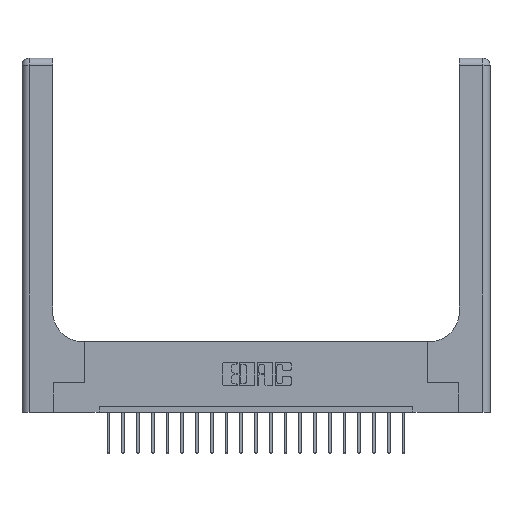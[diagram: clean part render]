
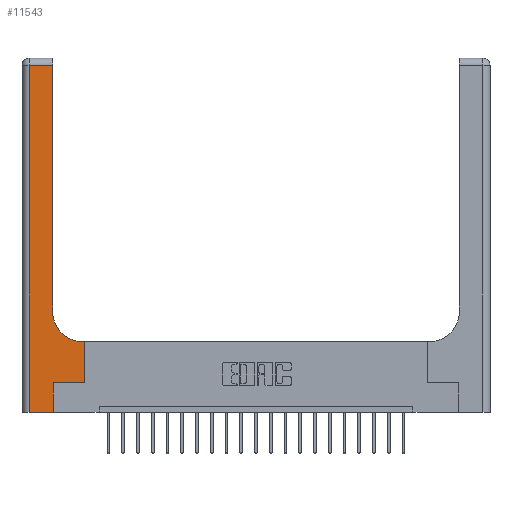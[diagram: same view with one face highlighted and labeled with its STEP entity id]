
A CAD part, top view. The second image highlights one B-rep face of the part: STEP entity #11543.
In plain terms, the highlighted planar face has unit normal (0, 0, 1).
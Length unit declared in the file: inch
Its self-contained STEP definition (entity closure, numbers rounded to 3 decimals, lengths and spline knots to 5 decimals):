
#405 = ORIENTED_EDGE ( 'NONE', *, *, #6993, .T. ) ;
#1041 = CARTESIAN_POINT ( 'NONE',  ( 0.26, 2.94, 0.37 ) ) ;
#1133 = EDGE_CURVE ( 'NONE', #8894, #18805, #10261, .T. ) ;
#1450 = VERTEX_POINT ( 'NONE', #1041 ) ;
#1686 = DIRECTION ( 'NONE',  ( 0., 1., 0. ) ) ;
#1790 = FACE_OUTER_BOUND ( 'NONE', #7415, .T. ) ;
#1892 = DIRECTION ( 'NONE',  ( 0., 0., -1. ) ) ;
#2078 = EDGE_CURVE ( 'NONE', #5481, #1450, #10321, .T. ) ;
#2083 = VECTOR ( 'NONE', #10715, 39.37008 ) ;
#2182 = EDGE_CURVE ( 'NONE', #18805, #15296, #10542, .T. ) ;
#2325 = LINE ( 'NONE', #15711, #11010 ) ;
#2401 = CARTESIAN_POINT ( 'NONE',  ( 0.26, 3., 0.37 ) ) ;
#2431 = LINE ( 'NONE', #17546, #16865 ) ;
#2942 = ORIENTED_EDGE ( 'NONE', *, *, #8634, .T. ) ;
#3044 = EDGE_CURVE ( 'NONE', #15296, #12000, #2431, .T. ) ;
#3555 = CARTESIAN_POINT ( 'NONE',  ( 0., 0., 0.37 ) ) ;
#3793 = ORIENTED_EDGE ( 'NONE', *, *, #3044, .T. ) ;
#4029 = CARTESIAN_POINT ( 'NONE',  ( 0.528, 0.6, 0.37 ) ) ;
#4092 = CARTESIAN_POINT ( 'NONE',  ( 0.06, 3., 0.37 ) ) ;
#4332 = EDGE_CURVE ( 'NONE', #12000, #19347, #2325, .T. ) ;
#5275 = DIRECTION ( 'NONE',  ( -1., 0., 0. ) ) ;
#5481 = VERTEX_POINT ( 'NONE', #11119 ) ;
#5564 = DIRECTION ( 'NONE',  ( 0., 1., 0. ) ) ;
#6457 = VECTOR ( 'NONE', #13951, 39.37008 ) ;
#6531 = EDGE_CURVE ( 'NONE', #18499, #8894, #13233, .T. ) ;
#6904 = AXIS2_PLACEMENT_3D ( 'NONE', #15158, #1892, #5275 ) ;
#6993 = EDGE_CURVE ( 'NONE', #1450, #12111, #10552, .T. ) ;
#7298 = DIRECTION ( 'NONE',  ( 1., 0., 0. ) ) ;
#7363 = VECTOR ( 'NONE', #1686, 39.37008 ) ;
#7415 = EDGE_LOOP ( 'NONE', ( #11265, #405, #20200, #7693, #12665, #9501, #3793, #12637, #2942 ) ) ;
#7639 = DIRECTION ( 'NONE',  ( 0., 1., 0. ) ) ;
#7693 = ORIENTED_EDGE ( 'NONE', *, *, #6531, .T. ) ;
#8293 = CARTESIAN_POINT ( 'NONE',  ( 0.06, 0., 0.37 ) ) ;
#8634 = EDGE_CURVE ( 'NONE', #19347, #5481, #20133, .T. ) ;
#8894 = VERTEX_POINT ( 'NONE', #12503 ) ;
#9143 = CARTESIAN_POINT ( 'NONE',  ( 0., 2.94, 0.37 ) ) ;
#9501 = ORIENTED_EDGE ( 'NONE', *, *, #2182, .T. ) ;
#10261 = LINE ( 'NONE', #16603, #7363 ) ;
#10321 = LINE ( 'NONE', #2401, #16769 ) ;
#10542 = LINE ( 'NONE', #15452, #11556 ) ;
#10552 = LINE ( 'NONE', #9143, #6457 ) ;
#10602 = LINE ( 'NONE', #4092, #2083 ) ;
#10715 = DIRECTION ( 'NONE',  ( 0., -1., 0. ) ) ;
#10984 = CARTESIAN_POINT ( 'NONE',  ( 0.06, 2.94, 0.37 ) ) ;
#11010 = VECTOR ( 'NONE', #17349, 39.37008 ) ;
#11082 = EDGE_CURVE ( 'NONE', #12111, #18499, #10602, .T. ) ;
#11119 = CARTESIAN_POINT ( 'NONE',  ( 0.26, 0.85, 0.37 ) ) ;
#11265 = ORIENTED_EDGE ( 'NONE', *, *, #2078, .T. ) ;
#11543 = ADVANCED_FACE ( 'NONE', ( #1790 ), #11896, .F. ) ;
#11556 = VECTOR ( 'NONE', #7298, 39.37008 ) ;
#11896 = PLANE ( 'NONE',  #6904 ) ;
#12000 = VERTEX_POINT ( 'NONE', #4029 ) ;
#12111 = VERTEX_POINT ( 'NONE', #10984 ) ;
#12503 = CARTESIAN_POINT ( 'NONE',  ( 0.265, 0., 0.37 ) ) ;
#12637 = ORIENTED_EDGE ( 'NONE', *, *, #4332, .T. ) ;
#12665 = ORIENTED_EDGE ( 'NONE', *, *, #1133, .T. ) ;
#13233 = LINE ( 'NONE', #3555, #16095 ) ;
#13951 = DIRECTION ( 'NONE',  ( -1., 0., 0. ) ) ;
#14907 = CARTESIAN_POINT ( 'NONE',  ( 0.51, 0.85, 0.37 ) ) ;
#14941 = AXIS2_PLACEMENT_3D ( 'NONE', #14907, #16345, #21349 ) ;
#15068 = CARTESIAN_POINT ( 'NONE',  ( 0.51, 0.6, 0.37 ) ) ;
#15158 = CARTESIAN_POINT ( 'NONE',  ( 0., 3., 0.37 ) ) ;
#15296 = VERTEX_POINT ( 'NONE', #18465 ) ;
#15452 = CARTESIAN_POINT ( 'NONE',  ( 0.265, 0.25, 0.37 ) ) ;
#15711 = CARTESIAN_POINT ( 'NONE',  ( 0.26, 0.6, 0.37 ) ) ;
#16095 = VECTOR ( 'NONE', #16512, 39.37008 ) ;
#16345 = DIRECTION ( 'NONE',  ( 0., 0., -1. ) ) ;
#16512 = DIRECTION ( 'NONE',  ( 1., 0., 0. ) ) ;
#16603 = CARTESIAN_POINT ( 'NONE',  ( 0.265, 0., 0.37 ) ) ;
#16769 = VECTOR ( 'NONE', #5564, 39.37008 ) ;
#16865 = VECTOR ( 'NONE', #7639, 39.37008 ) ;
#17349 = DIRECTION ( 'NONE',  ( -1., 0., 0. ) ) ;
#17546 = CARTESIAN_POINT ( 'NONE',  ( 0.528, 0.25, 0.37 ) ) ;
#18037 = CARTESIAN_POINT ( 'NONE',  ( 0.265, 0.25, 0.37 ) ) ;
#18465 = CARTESIAN_POINT ( 'NONE',  ( 0.528, 0.25, 0.37 ) ) ;
#18499 = VERTEX_POINT ( 'NONE', #8293 ) ;
#18805 = VERTEX_POINT ( 'NONE', #18037 ) ;
#19347 = VERTEX_POINT ( 'NONE', #15068 ) ;
#20133 = CIRCLE ( 'NONE', #14941, 0.25 ) ;
#20200 = ORIENTED_EDGE ( 'NONE', *, *, #11082, .T. ) ;
#21349 = DIRECTION ( 'NONE',  ( 1., 0., 0. ) ) ;
